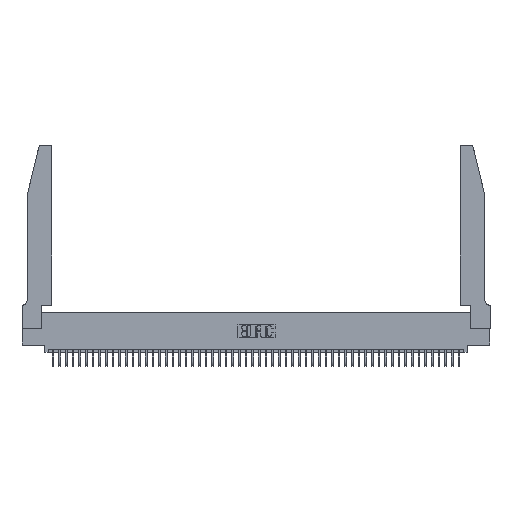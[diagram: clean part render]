
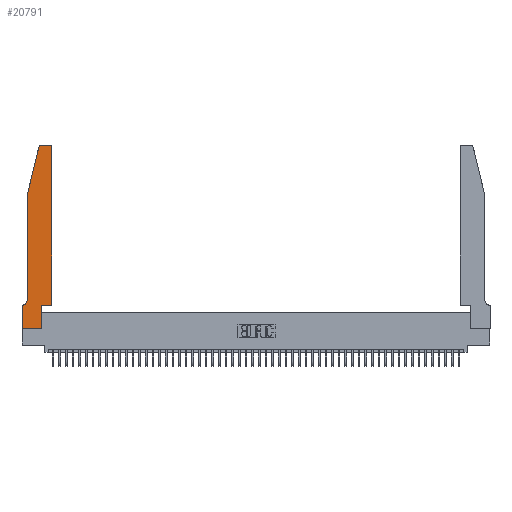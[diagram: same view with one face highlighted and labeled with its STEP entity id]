
A CAD part, top view. The second image highlights one B-rep face of the part: STEP entity #20791.
In plain terms, the highlighted planar face has unit normal (0, 0, 1).
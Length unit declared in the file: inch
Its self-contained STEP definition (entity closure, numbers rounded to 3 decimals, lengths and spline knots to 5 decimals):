
#462 = LINE ( 'NONE', #43482, #20896 ) ;
#782 = CARTESIAN_POINT ( 'NONE',  ( 0.2605, 2.75, 0.37 ) ) ;
#1577 = CARTESIAN_POINT ( 'NONE',  ( 0.4505, 2.72, 0.37 ) ) ;
#1785 = CARTESIAN_POINT ( 'NONE',  ( 0., 0., 0.37 ) ) ;
#2087 = DIRECTION ( 'NONE',  ( 1., 0., 0. ) ) ;
#2096 = ORIENTED_EDGE ( 'NONE', *, *, #26289, .T. ) ;
#3540 = AXIS2_PLACEMENT_3D ( 'NONE', #34571, #10217, #38598 ) ;
#3796 = EDGE_CURVE ( 'NONE', #30854, #25037, #23414, .T. ) ;
#4414 = ORIENTED_EDGE ( 'NONE', *, *, #24123, .T. ) ;
#5491 = VECTOR ( 'NONE', #12242, 39.37008 ) ;
#6094 = LINE ( 'NONE', #48020, #38522 ) ;
#6192 = EDGE_LOOP ( 'NONE', ( #9053, #34462, #24459, #32020, #46546, #4414, #39296, #52058, #35110, #2096, #8824, #46332 ) ) ;
#8271 = CARTESIAN_POINT ( 'NONE',  ( 0.0755, 2., 0.37 ) ) ;
#8824 = ORIENTED_EDGE ( 'NONE', *, *, #33640, .T. ) ;
#9053 = ORIENTED_EDGE ( 'NONE', *, *, #3796, .T. ) ;
#9582 = VERTEX_POINT ( 'NONE', #1577 ) ;
#9978 = LINE ( 'NONE', #25530, #30328 ) ;
#10202 = DIRECTION ( 'NONE',  ( 0., -1., 0. ) ) ;
#10217 = DIRECTION ( 'NONE',  ( 0., 0., 1. ) ) ;
#11080 = EDGE_CURVE ( 'NONE', #29739, #17163, #48649, .T. ) ;
#12242 = DIRECTION ( 'NONE',  ( 0., -1., 0. ) ) ;
#12485 = VERTEX_POINT ( 'NONE', #13533 ) ;
#13401 = EDGE_CURVE ( 'NONE', #17163, #34413, #23149, .T. ) ;
#13533 = CARTESIAN_POINT ( 'NONE',  ( 0.2865, 0., 0.37 ) ) ;
#13662 = CARTESIAN_POINT ( 'NONE',  ( 0.0755, 0.35, 0.37 ) ) ;
#13814 = VECTOR ( 'NONE', #29266, 39.37008 ) ;
#14916 = DIRECTION ( 'NONE',  ( -0.239, -0.971, 0. ) ) ;
#14920 = CARTESIAN_POINT ( 'NONE',  ( 0., 0., 0.37 ) ) ;
#15386 = PLANE ( 'NONE',  #36981 ) ;
#17163 = VERTEX_POINT ( 'NONE', #47195 ) ;
#17717 = VECTOR ( 'NONE', #10202, 39.37008 ) ;
#18150 = CARTESIAN_POINT ( 'NONE',  ( 0.284, 2.75, 0.37 ) ) ;
#19231 = CARTESIAN_POINT ( 'NONE',  ( 0.0755, 2., 0.37 ) ) ;
#19500 = DIRECTION ( 'NONE',  ( 0., 0., 1. ) ) ;
#19543 = CARTESIAN_POINT ( 'NONE',  ( 0.0055, 0.42, 0.37 ) ) ;
#20100 = CIRCLE ( 'NONE', #3540, 0.03 ) ;
#20791 = ADVANCED_FACE ( 'NONE', ( #47887 ), #15386, .T. ) ;
#20896 = VECTOR ( 'NONE', #47521, 39.37008 ) ;
#21262 = VERTEX_POINT ( 'NONE', #22642 ) ;
#22337 = CARTESIAN_POINT ( 'NONE',  ( 0.2865, 0.35, 0.37 ) ) ;
#22626 = CARTESIAN_POINT ( 'NONE',  ( 0.4505, 0.35, 0.37 ) ) ;
#22642 = CARTESIAN_POINT ( 'NONE',  ( 0., 0.35, 0.37 ) ) ;
#23149 = CIRCLE ( 'NONE', #48249, 0.07 ) ;
#23414 = LINE ( 'NONE', #782, #13814 ) ;
#23527 = EDGE_CURVE ( 'NONE', #42627, #12485, #28654, .T. ) ;
#23630 = DIRECTION ( 'NONE',  ( -1., 0., 0. ) ) ;
#24123 = EDGE_CURVE ( 'NONE', #34413, #21262, #44467, .T. ) ;
#24244 = VECTOR ( 'NONE', #14916, 39.37008 ) ;
#24459 = ORIENTED_EDGE ( 'NONE', *, *, #27313, .T. ) ;
#25037 = VERTEX_POINT ( 'NONE', #18150 ) ;
#25530 = CARTESIAN_POINT ( 'NONE',  ( 0.4505, 0.35, 0.37 ) ) ;
#25680 = CIRCLE ( 'NONE', #30428, 0.03 ) ;
#26289 = EDGE_CURVE ( 'NONE', #51701, #50341, #9978, .T. ) ;
#26499 = DIRECTION ( 'NONE',  ( 0., 0., 1. ) ) ;
#27313 = EDGE_CURVE ( 'NONE', #45179, #29739, #45684, .T. ) ;
#27909 = DIRECTION ( 'NONE',  ( 0., 1., 0. ) ) ;
#28543 = LINE ( 'NONE', #46495, #17717 ) ;
#28654 = LINE ( 'NONE', #1785, #39397 ) ;
#29266 = DIRECTION ( 'NONE',  ( -1., 0., 0. ) ) ;
#29571 = DIRECTION ( 'NONE',  ( 1., 0., 0. ) ) ;
#29739 = VERTEX_POINT ( 'NONE', #8271 ) ;
#30056 = EDGE_CURVE ( 'NONE', #9582, #30854, #20100, .T. ) ;
#30328 = VECTOR ( 'NONE', #29571, 39.37008 ) ;
#30428 = AXIS2_PLACEMENT_3D ( 'NONE', #50657, #26499, #2087 ) ;
#30854 = VERTEX_POINT ( 'NONE', #39231 ) ;
#32020 = ORIENTED_EDGE ( 'NONE', *, *, #11080, .T. ) ;
#32476 = VECTOR ( 'NONE', #50127, 39.37008 ) ;
#33640 = EDGE_CURVE ( 'NONE', #50341, #9582, #6094, .T. ) ;
#34413 = VERTEX_POINT ( 'NONE', #34937 ) ;
#34462 = ORIENTED_EDGE ( 'NONE', *, *, #40578, .T. ) ;
#34571 = CARTESIAN_POINT ( 'NONE',  ( 0.4205, 2.72, 0.37 ) ) ;
#34937 = CARTESIAN_POINT ( 'NONE',  ( 0.0055, 0.35, 0.37 ) ) ;
#35110 = ORIENTED_EDGE ( 'NONE', *, *, #43615, .T. ) ;
#36981 = AXIS2_PLACEMENT_3D ( 'NONE', #43720, #19500, #47761 ) ;
#38522 = VECTOR ( 'NONE', #27909, 39.37008 ) ;
#38598 = DIRECTION ( 'NONE',  ( 1., 0., 0. ) ) ;
#39231 = CARTESIAN_POINT ( 'NONE',  ( 0.4205, 2.75, 0.37 ) ) ;
#39296 = ORIENTED_EDGE ( 'NONE', *, *, #51704, .T. ) ;
#39397 = VECTOR ( 'NONE', #42433, 39.37008 ) ;
#40578 = EDGE_CURVE ( 'NONE', #25037, #45179, #25680, .T. ) ;
#40605 = CARTESIAN_POINT ( 'NONE',  ( 0.0755, 2., 0.37 ) ) ;
#42433 = DIRECTION ( 'NONE',  ( 1., 0., 0. ) ) ;
#42627 = VERTEX_POINT ( 'NONE', #14920 ) ;
#43482 = CARTESIAN_POINT ( 'NONE',  ( 0.2865, 0.35, 0.37 ) ) ;
#43615 = EDGE_CURVE ( 'NONE', #12485, #51701, #462, .T. ) ;
#43720 = CARTESIAN_POINT ( 'NONE',  ( 0., 0.35, 0.37 ) ) ;
#44467 = LINE ( 'NONE', #13662, #32476 ) ;
#45179 = VERTEX_POINT ( 'NONE', #50201 ) ;
#45684 = LINE ( 'NONE', #19231, #24244 ) ;
#46332 = ORIENTED_EDGE ( 'NONE', *, *, #30056, .T. ) ;
#46495 = CARTESIAN_POINT ( 'NONE',  ( 0., 0., 0.37 ) ) ;
#46546 = ORIENTED_EDGE ( 'NONE', *, *, #13401, .T. ) ;
#47195 = CARTESIAN_POINT ( 'NONE',  ( 0.0755, 0.42, 0.37 ) ) ;
#47521 = DIRECTION ( 'NONE',  ( 0., 1., 0. ) ) ;
#47761 = DIRECTION ( 'NONE',  ( 1., 0., 0. ) ) ;
#47798 = DIRECTION ( 'NONE',  ( 0., 0., -1. ) ) ;
#47887 = FACE_OUTER_BOUND ( 'NONE', #6192, .T. ) ;
#48020 = CARTESIAN_POINT ( 'NONE',  ( 0.4505, 0.35, 0.37 ) ) ;
#48249 = AXIS2_PLACEMENT_3D ( 'NONE', #19543, #47798, #23630 ) ;
#48649 = LINE ( 'NONE', #40605, #5491 ) ;
#50127 = DIRECTION ( 'NONE',  ( -1., 0., 0. ) ) ;
#50201 = CARTESIAN_POINT ( 'NONE',  ( 0.25487, 2.72718, 0.37 ) ) ;
#50341 = VERTEX_POINT ( 'NONE', #22626 ) ;
#50657 = CARTESIAN_POINT ( 'NONE',  ( 0.284, 2.72, 0.37 ) ) ;
#51701 = VERTEX_POINT ( 'NONE', #22337 ) ;
#51704 = EDGE_CURVE ( 'NONE', #21262, #42627, #28543, .T. ) ;
#52058 = ORIENTED_EDGE ( 'NONE', *, *, #23527, .T. ) ;
